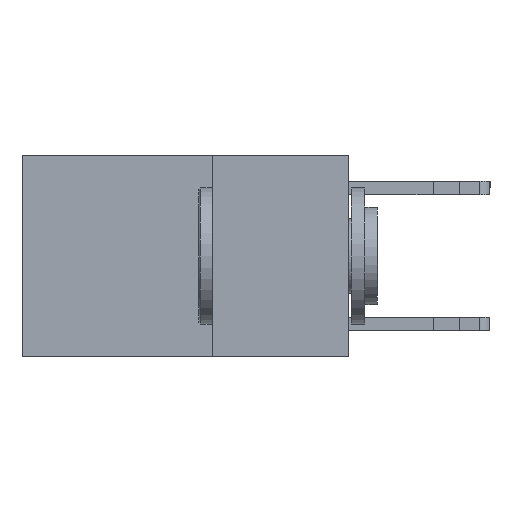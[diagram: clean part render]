
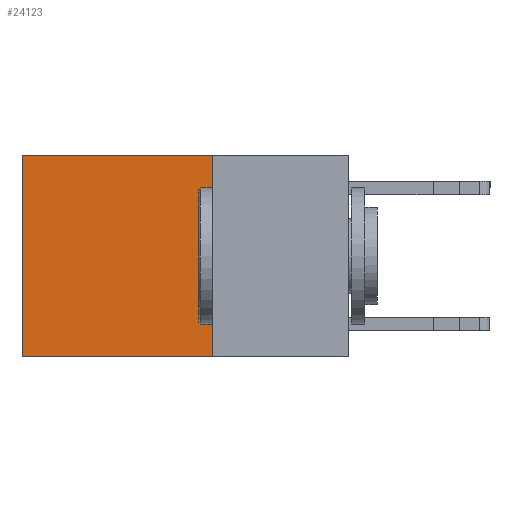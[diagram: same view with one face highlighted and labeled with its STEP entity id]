
A CAD part, left-side view. The second image highlights one B-rep face of the part: STEP entity #24123.
In plain terms, the highlighted planar face has unit normal (-1, 0, 0).
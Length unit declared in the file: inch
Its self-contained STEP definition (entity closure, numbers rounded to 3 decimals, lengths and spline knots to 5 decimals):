
#594 = LINE ( 'NONE', #19387, #18966 ) ;
#937 = VERTEX_POINT ( 'NONE', #12250 ) ;
#3096 = VECTOR ( 'NONE', #16407, 39.37008 ) ;
#3472 = ORIENTED_EDGE ( 'NONE', *, *, #21588, .T. ) ;
#3783 = VERTEX_POINT ( 'NONE', #8986 ) ;
#6339 = VERTEX_POINT ( 'NONE', #22567 ) ;
#6567 = DIRECTION ( 'NONE',  ( 0., 0., -1. ) ) ;
#7189 = EDGE_LOOP ( 'NONE', ( #3472, #12147, #11214, #16756 ) ) ;
#8032 = DIRECTION ( 'NONE',  ( 0., 1., 0. ) ) ;
#8680 = DIRECTION ( 'NONE',  ( 0., 1., 0. ) ) ;
#8887 = CARTESIAN_POINT ( 'NONE',  ( 0.2625, 0.6, 0. ) ) ;
#8986 = CARTESIAN_POINT ( 'NONE',  ( 0.2625, 0.25, 0. ) ) ;
#10383 = LINE ( 'NONE', #17556, #15390 ) ;
#10738 = LINE ( 'NONE', #8887, #3096 ) ;
#11048 = AXIS2_PLACEMENT_3D ( 'NONE', #22770, #20918, #21523 ) ;
#11214 = ORIENTED_EDGE ( 'NONE', *, *, #15337, .F. ) ;
#12147 = ORIENTED_EDGE ( 'NONE', *, *, #15810, .F. ) ;
#12250 = CARTESIAN_POINT ( 'NONE',  ( 0.2625, 0.6, -0.37 ) ) ;
#12750 = LINE ( 'NONE', #24102, #12995 ) ;
#12995 = VECTOR ( 'NONE', #8680, 39.37008 ) ;
#15232 = PLANE ( 'NONE',  #11048 ) ;
#15337 = EDGE_CURVE ( 'NONE', #3783, #6339, #10383, .T. ) ;
#15390 = VECTOR ( 'NONE', #6567, 39.37008 ) ;
#15810 = EDGE_CURVE ( 'NONE', #6339, #937, #594, .T. ) ;
#16407 = DIRECTION ( 'NONE',  ( 0., 0., -1. ) ) ;
#16756 = ORIENTED_EDGE ( 'NONE', *, *, #21091, .T. ) ;
#17087 = FACE_OUTER_BOUND ( 'NONE', #7189, .T. ) ;
#17556 = CARTESIAN_POINT ( 'NONE',  ( 0.2625, 0.25, 0. ) ) ;
#18966 = VECTOR ( 'NONE', #8032, 39.37008 ) ;
#19387 = CARTESIAN_POINT ( 'NONE',  ( 0.2625, 0.25, -0.37 ) ) ;
#20546 = CARTESIAN_POINT ( 'NONE',  ( 0.2625, 0.6, 0. ) ) ;
#20918 = DIRECTION ( 'NONE',  ( 1., 0., 0. ) ) ;
#21091 = EDGE_CURVE ( 'NONE', #3783, #23963, #12750, .T. ) ;
#21523 = DIRECTION ( 'NONE',  ( 0., 0., -1. ) ) ;
#21588 = EDGE_CURVE ( 'NONE', #23963, #937, #10738, .T. ) ;
#22567 = CARTESIAN_POINT ( 'NONE',  ( 0.2625, 0.25, -0.37 ) ) ;
#22770 = CARTESIAN_POINT ( 'NONE',  ( 0.2625, 0.25, 0. ) ) ;
#23963 = VERTEX_POINT ( 'NONE', #20546 ) ;
#24102 = CARTESIAN_POINT ( 'NONE',  ( 0.2625, 0.25, 0. ) ) ;
#24123 = ADVANCED_FACE ( 'NONE', ( #17087 ), #15232, .F. ) ;
